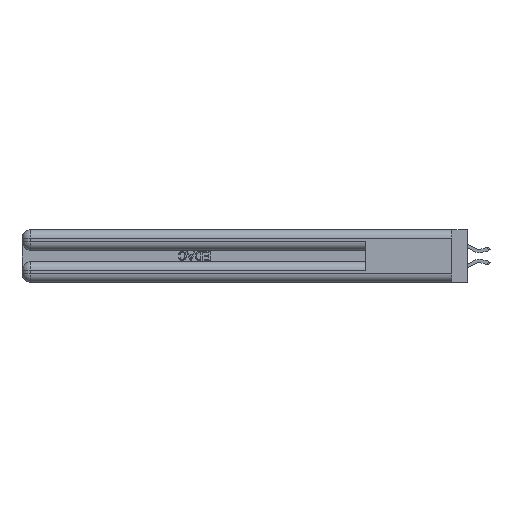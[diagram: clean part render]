
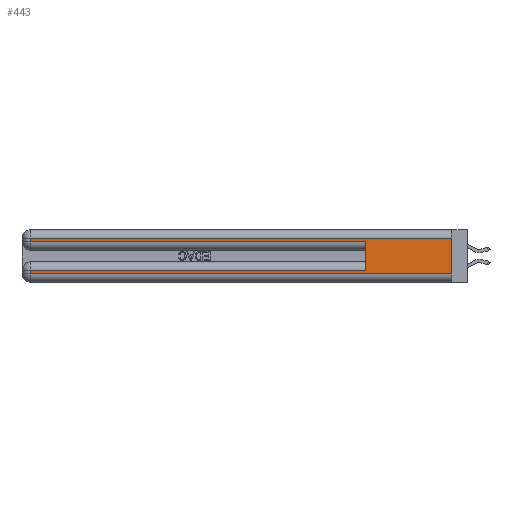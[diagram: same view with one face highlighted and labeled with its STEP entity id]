
A CAD part, left-side view. The second image highlights one B-rep face of the part: STEP entity #443.
In plain terms, the highlighted planar face has unit normal (-1, 0, 0).
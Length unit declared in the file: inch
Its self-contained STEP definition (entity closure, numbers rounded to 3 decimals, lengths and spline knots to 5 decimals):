
#443 = ADVANCED_FACE ( 'NONE', ( #36171 ), #18013, .F. ) ;
#650 = CARTESIAN_POINT ( 'NONE',  ( 0., 2.94, 0.285 ) ) ;
#2215 = ORIENTED_EDGE ( 'NONE', *, *, #13385, .T. ) ;
#2438 = CARTESIAN_POINT ( 'NONE',  ( 0., 2.94, 0.085 ) ) ;
#2797 = EDGE_LOOP ( 'NONE', ( #12383, #24115, #2215, #31525, #14794, #22429, #14330, #20182 ) ) ;
#3818 = CARTESIAN_POINT ( 'NONE',  ( 0., 0.6, 0.285 ) ) ;
#4814 = DIRECTION ( 'NONE',  ( 0., -1., 0. ) ) ;
#4936 = CARTESIAN_POINT ( 'NONE',  ( 0., 0., 0.06 ) ) ;
#5908 = CARTESIAN_POINT ( 'NONE',  ( 0., 2.94, 0.37 ) ) ;
#6647 = CARTESIAN_POINT ( 'NONE',  ( 0., 0., 0.085 ) ) ;
#6844 = AXIS2_PLACEMENT_3D ( 'NONE', #18143, #32762, #8205 ) ;
#7252 = DIRECTION ( 'NONE',  ( 0., 0., -1. ) ) ;
#7760 = EDGE_CURVE ( 'NONE', #38867, #21780, #14448, .T. ) ;
#8205 = DIRECTION ( 'NONE',  ( 0., 0., -1. ) ) ;
#8533 = LINE ( 'NONE', #21164, #34965 ) ;
#9241 = VERTEX_POINT ( 'NONE', #28625 ) ;
#10628 = EDGE_CURVE ( 'NONE', #21592, #17790, #17945, .T. ) ;
#11030 = DIRECTION ( 'NONE',  ( 0., -1., 0. ) ) ;
#11316 = LINE ( 'NONE', #26814, #33519 ) ;
#11882 = DIRECTION ( 'NONE',  ( 0., 0., -1. ) ) ;
#12383 = ORIENTED_EDGE ( 'NONE', *, *, #32119, .F. ) ;
#12938 = CARTESIAN_POINT ( 'NONE',  ( 0., 2.94, 0.31 ) ) ;
#13385 = EDGE_CURVE ( 'NONE', #17066, #38867, #11316, .T. ) ;
#14330 = ORIENTED_EDGE ( 'NONE', *, *, #10628, .T. ) ;
#14448 = LINE ( 'NONE', #22858, #14907 ) ;
#14794 = ORIENTED_EDGE ( 'NONE', *, *, #36492, .F. ) ;
#14891 = VECTOR ( 'NONE', #27185, 39.37008 ) ;
#14907 = VECTOR ( 'NONE', #4814, 39.37008 ) ;
#15505 = VERTEX_POINT ( 'NONE', #15636 ) ;
#15636 = CARTESIAN_POINT ( 'NONE',  ( 0., 0., 0.06 ) ) ;
#17066 = VERTEX_POINT ( 'NONE', #12938 ) ;
#17790 = VERTEX_POINT ( 'NONE', #30619 ) ;
#17817 = EDGE_CURVE ( 'NONE', #37647, #21592, #27110, .T. ) ;
#17945 = LINE ( 'NONE', #5908, #26401 ) ;
#18013 = PLANE ( 'NONE',  #6844 ) ;
#18143 = CARTESIAN_POINT ( 'NONE',  ( 0., 0., 0.37 ) ) ;
#18749 = DIRECTION ( 'NONE',  ( 0., 0., 1. ) ) ;
#19701 = EDGE_CURVE ( 'NONE', #17790, #15505, #31773, .T. ) ;
#20182 = ORIENTED_EDGE ( 'NONE', *, *, #19701, .T. ) ;
#20418 = CARTESIAN_POINT ( 'NONE',  ( 0., 0., 0.31 ) ) ;
#21164 = CARTESIAN_POINT ( 'NONE',  ( 0., 0., 0.37 ) ) ;
#21592 = VERTEX_POINT ( 'NONE', #2438 ) ;
#21780 = VERTEX_POINT ( 'NONE', #3818 ) ;
#21816 = CARTESIAN_POINT ( 'NONE',  ( 0., 0.6, 0.085 ) ) ;
#21859 = LINE ( 'NONE', #33854, #31378 ) ;
#22267 = VECTOR ( 'NONE', #29686, 39.37008 ) ;
#22429 = ORIENTED_EDGE ( 'NONE', *, *, #17817, .T. ) ;
#22858 = CARTESIAN_POINT ( 'NONE',  ( 0., 0., 0.285 ) ) ;
#23699 = VECTOR ( 'NONE', #11030, 39.37008 ) ;
#24115 = ORIENTED_EDGE ( 'NONE', *, *, #37403, .T. ) ;
#26401 = VECTOR ( 'NONE', #7252, 39.37008 ) ;
#26814 = CARTESIAN_POINT ( 'NONE',  ( 0., 2.94, 0.37 ) ) ;
#27110 = LINE ( 'NONE', #6647, #14891 ) ;
#27185 = DIRECTION ( 'NONE',  ( 0., 1., 0. ) ) ;
#28625 = CARTESIAN_POINT ( 'NONE',  ( 0., 0., 0.31 ) ) ;
#29686 = DIRECTION ( 'NONE',  ( 0., 1., 0. ) ) ;
#30619 = CARTESIAN_POINT ( 'NONE',  ( 0., 2.94, 0.06 ) ) ;
#31322 = LINE ( 'NONE', #20418, #22267 ) ;
#31378 = VECTOR ( 'NONE', #18749, 39.37008 ) ;
#31525 = ORIENTED_EDGE ( 'NONE', *, *, #7760, .T. ) ;
#31773 = LINE ( 'NONE', #4936, #23699 ) ;
#32119 = EDGE_CURVE ( 'NONE', #9241, #15505, #8533, .T. ) ;
#32762 = DIRECTION ( 'NONE',  ( 1., 0., 0. ) ) ;
#33519 = VECTOR ( 'NONE', #36020, 39.37008 ) ;
#33854 = CARTESIAN_POINT ( 'NONE',  ( 0., 0.6, 0.145 ) ) ;
#34965 = VECTOR ( 'NONE', #11882, 39.37008 ) ;
#36020 = DIRECTION ( 'NONE',  ( 0., 0., -1. ) ) ;
#36171 = FACE_OUTER_BOUND ( 'NONE', #2797, .T. ) ;
#36492 = EDGE_CURVE ( 'NONE', #37647, #21780, #21859, .T. ) ;
#37403 = EDGE_CURVE ( 'NONE', #9241, #17066, #31322, .T. ) ;
#37647 = VERTEX_POINT ( 'NONE', #21816 ) ;
#38867 = VERTEX_POINT ( 'NONE', #650 ) ;
